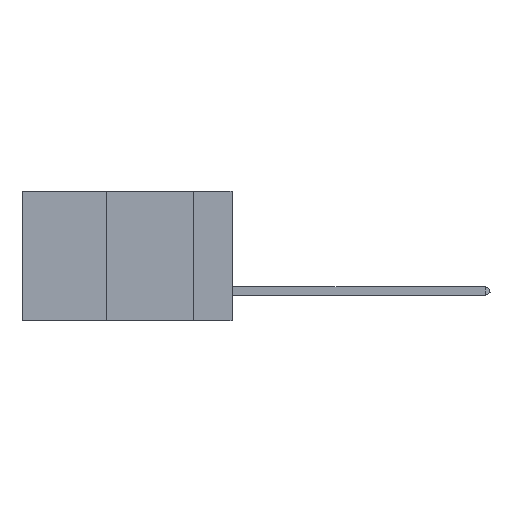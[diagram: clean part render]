
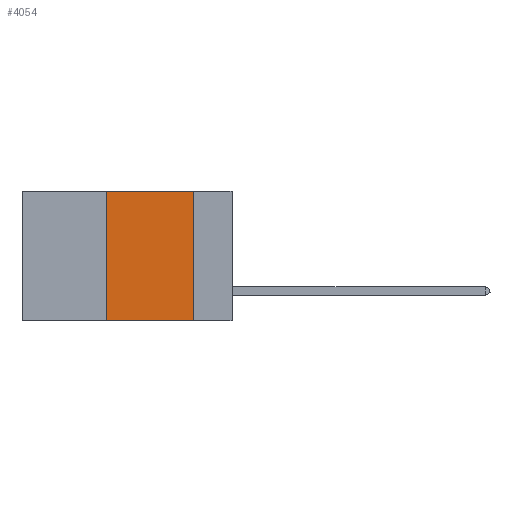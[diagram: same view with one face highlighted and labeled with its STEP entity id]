
A CAD part, left-side view. The second image highlights one B-rep face of the part: STEP entity #4054.
In plain terms, the highlighted planar face has unit normal (-1, 0, 0).
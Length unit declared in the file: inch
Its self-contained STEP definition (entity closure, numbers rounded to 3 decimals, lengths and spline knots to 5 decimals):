
#816 = CARTESIAN_POINT ( 'NONE',  ( 0., 0.11, 0. ) ) ;
#832 = EDGE_CURVE ( 'NONE', #6337, #4059, #2295, .T. ) ;
#891 = CARTESIAN_POINT ( 'NONE',  ( 0., 0.36, -0.37 ) ) ;
#1029 = VECTOR ( 'NONE', #11307, 39.37008 ) ;
#1664 = DIRECTION ( 'NONE',  ( 1., 0., 0. ) ) ;
#1773 = VECTOR ( 'NONE', #1787, 39.37008 ) ;
#1787 = DIRECTION ( 'NONE',  ( 0., -1., 0. ) ) ;
#2020 = LINE ( 'NONE', #816, #12675 ) ;
#2295 = LINE ( 'NONE', #10543, #11079 ) ;
#3033 = LINE ( 'NONE', #8917, #1029 ) ;
#3882 = ORIENTED_EDGE ( 'NONE', *, *, #10342, .F. ) ;
#4054 = ADVANCED_FACE ( 'NONE', ( #7020 ), #12033, .F. ) ;
#4059 = VERTEX_POINT ( 'NONE', #4099 ) ;
#4099 = CARTESIAN_POINT ( 'NONE',  ( 0., 0.11, 0. ) ) ;
#4599 = EDGE_CURVE ( 'NONE', #8317, #11864, #8109, .T. ) ;
#5557 = DIRECTION ( 'NONE',  ( 0., 0., -1. ) ) ;
#6337 = VERTEX_POINT ( 'NONE', #6611 ) ;
#6611 = CARTESIAN_POINT ( 'NONE',  ( 0., 0.36, 0. ) ) ;
#7020 = FACE_OUTER_BOUND ( 'NONE', #10110, .T. ) ;
#7315 = EDGE_CURVE ( 'NONE', #8317, #6337, #3033, .T. ) ;
#8109 = LINE ( 'NONE', #13268, #1773 ) ;
#8317 = VERTEX_POINT ( 'NONE', #891 ) ;
#8544 = CARTESIAN_POINT ( 'NONE',  ( 0., 0.6, 0. ) ) ;
#8917 = CARTESIAN_POINT ( 'NONE',  ( 0., 0.36, 0. ) ) ;
#8931 = CARTESIAN_POINT ( 'NONE',  ( 0., 0.11, -0.37 ) ) ;
#9693 = DIRECTION ( 'NONE',  ( 0., 0., -1. ) ) ;
#10110 = EDGE_LOOP ( 'NONE', ( #3882, #14650, #11005, #10533 ) ) ;
#10342 = EDGE_CURVE ( 'NONE', #4059, #11864, #2020, .T. ) ;
#10533 = ORIENTED_EDGE ( 'NONE', *, *, #4599, .T. ) ;
#10543 = CARTESIAN_POINT ( 'NONE',  ( 0., 0.6, 0. ) ) ;
#11005 = ORIENTED_EDGE ( 'NONE', *, *, #7315, .F. ) ;
#11079 = VECTOR ( 'NONE', #11778, 39.37008 ) ;
#11307 = DIRECTION ( 'NONE',  ( 0., 0., 1. ) ) ;
#11778 = DIRECTION ( 'NONE',  ( 0., -1., 0. ) ) ;
#11864 = VERTEX_POINT ( 'NONE', #8931 ) ;
#12033 = PLANE ( 'NONE',  #12301 ) ;
#12301 = AXIS2_PLACEMENT_3D ( 'NONE', #8544, #1664, #9693 ) ;
#12675 = VECTOR ( 'NONE', #5557, 39.37008 ) ;
#13268 = CARTESIAN_POINT ( 'NONE',  ( 0., 0.6, -0.37 ) ) ;
#14650 = ORIENTED_EDGE ( 'NONE', *, *, #832, .F. ) ;
